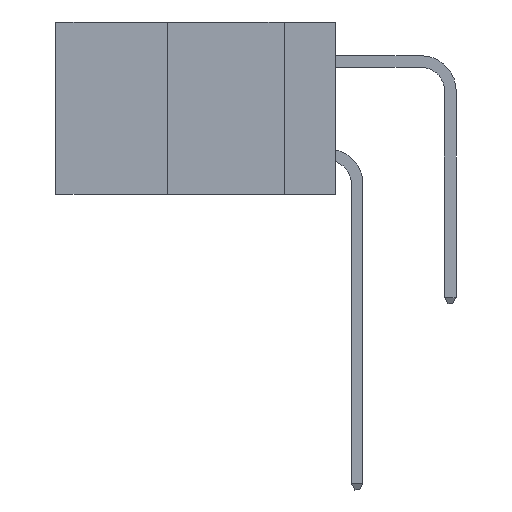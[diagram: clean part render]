
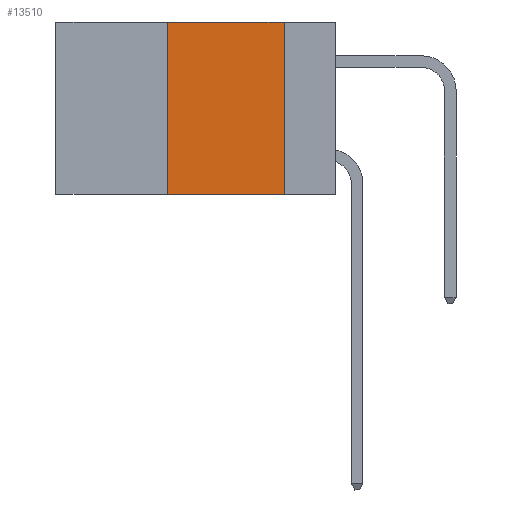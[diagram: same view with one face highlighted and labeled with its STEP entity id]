
A CAD part, left-side view. The second image highlights one B-rep face of the part: STEP entity #13510.
In plain terms, the highlighted planar face has unit normal (-1, 0, 0).
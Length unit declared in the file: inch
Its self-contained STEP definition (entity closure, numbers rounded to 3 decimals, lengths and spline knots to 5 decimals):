
#29 = LINE ( 'NONE', #14468, #2614 ) ;
#628 = PLANE ( 'NONE',  #5633 ) ;
#2058 = DIRECTION ( 'NONE',  ( 0., 0., -1. ) ) ;
#2606 = ORIENTED_EDGE ( 'NONE', *, *, #3038, .F. ) ;
#2614 = VECTOR ( 'NONE', #2058, 39.37008 ) ;
#3027 = VERTEX_POINT ( 'NONE', #13175 ) ;
#3038 = EDGE_CURVE ( 'NONE', #13734, #9009, #3757, .T. ) ;
#3497 = VECTOR ( 'NONE', #11480, 39.37008 ) ;
#3757 = LINE ( 'NONE', #11152, #6799 ) ;
#5581 = CARTESIAN_POINT ( 'NONE',  ( 0., 0.36, -0.37 ) ) ;
#5633 = AXIS2_PLACEMENT_3D ( 'NONE', #10836, #14199, #7437 ) ;
#5691 = EDGE_LOOP ( 'NONE', ( #6474, #12727, #2606, #14127 ) ) ;
#5866 = FACE_OUTER_BOUND ( 'NONE', #5691, .T. ) ;
#6361 = EDGE_CURVE ( 'NONE', #13734, #3027, #12912, .T. ) ;
#6474 = ORIENTED_EDGE ( 'NONE', *, *, #9125, .F. ) ;
#6799 = VECTOR ( 'NONE', #8863, 39.37008 ) ;
#7116 = VECTOR ( 'NONE', #9971, 39.37008 ) ;
#7437 = DIRECTION ( 'NONE',  ( 0., 0., -1. ) ) ;
#8863 = DIRECTION ( 'NONE',  ( 0., 0., 1. ) ) ;
#9009 = VERTEX_POINT ( 'NONE', #9792 ) ;
#9125 = EDGE_CURVE ( 'NONE', #11929, #3027, #29, .T. ) ;
#9792 = CARTESIAN_POINT ( 'NONE',  ( 0., 0.36, 0. ) ) ;
#9918 = CARTESIAN_POINT ( 'NONE',  ( 0., 0.6, 0. ) ) ;
#9971 = DIRECTION ( 'NONE',  ( 0., -1., 0. ) ) ;
#10836 = CARTESIAN_POINT ( 'NONE',  ( 0., 0.6, 0. ) ) ;
#10886 = LINE ( 'NONE', #9918, #7116 ) ;
#11152 = CARTESIAN_POINT ( 'NONE',  ( 0., 0.36, 0. ) ) ;
#11348 = CARTESIAN_POINT ( 'NONE',  ( 0., 0.11, 0. ) ) ;
#11480 = DIRECTION ( 'NONE',  ( 0., -1., 0. ) ) ;
#11929 = VERTEX_POINT ( 'NONE', #11348 ) ;
#12727 = ORIENTED_EDGE ( 'NONE', *, *, #14254, .F. ) ;
#12912 = LINE ( 'NONE', #13730, #3497 ) ;
#13175 = CARTESIAN_POINT ( 'NONE',  ( 0., 0.11, -0.37 ) ) ;
#13510 = ADVANCED_FACE ( 'NONE', ( #5866 ), #628, .F. ) ;
#13730 = CARTESIAN_POINT ( 'NONE',  ( 0., 0.6, -0.37 ) ) ;
#13734 = VERTEX_POINT ( 'NONE', #5581 ) ;
#14127 = ORIENTED_EDGE ( 'NONE', *, *, #6361, .T. ) ;
#14199 = DIRECTION ( 'NONE',  ( 1., 0., 0. ) ) ;
#14254 = EDGE_CURVE ( 'NONE', #9009, #11929, #10886, .T. ) ;
#14468 = CARTESIAN_POINT ( 'NONE',  ( 0., 0.11, 0. ) ) ;
